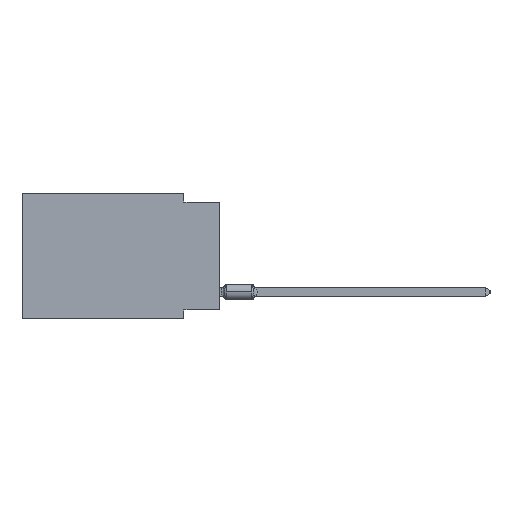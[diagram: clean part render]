
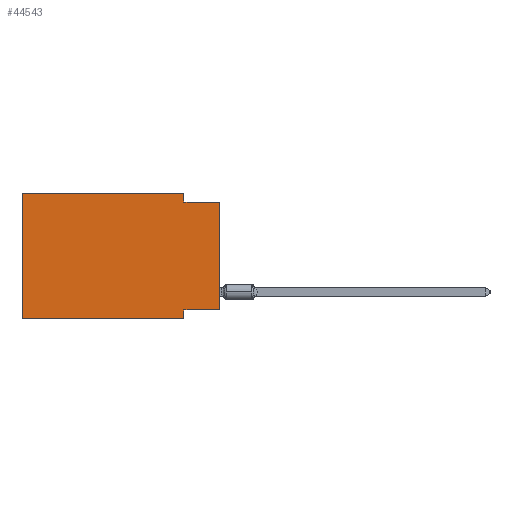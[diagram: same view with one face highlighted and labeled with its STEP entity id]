
A CAD part, left-side view. The second image highlights one B-rep face of the part: STEP entity #44543.
In plain terms, the highlighted planar face has unit normal (-1, 0, 0).
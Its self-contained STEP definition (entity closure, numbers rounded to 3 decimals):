
#1589 = VERTEX_POINT ( 'NONE', #3762 ) ;
#2478 = EDGE_CURVE ( 'NONE', #48055, #7422, #28816, .T. ) ;
#3762 = CARTESIAN_POINT ( 'NONE',  ( 0., 2.54, -8.255 ) ) ;
#4447 = EDGE_CURVE ( 'NONE', #39297, #37166, #8983, .T. ) ;
#7377 = CARTESIAN_POINT ( 'NONE',  ( 0., 2.54, -0.635 ) ) ;
#7422 = VERTEX_POINT ( 'NONE', #7377 ) ;
#7778 = DIRECTION ( 'NONE',  ( 0., -1., 0. ) ) ;
#7855 = ORIENTED_EDGE ( 'NONE', *, *, #27830, .T. ) ;
#7865 = CARTESIAN_POINT ( 'NONE',  ( 0., 0., 0. ) ) ;
#8552 = CARTESIAN_POINT ( 'NONE',  ( 0., 2.54, 0. ) ) ;
#8983 = LINE ( 'NONE', #50139, #48166 ) ;
#10203 = EDGE_CURVE ( 'NONE', #26647, #22648, #23977, .T. ) ;
#10567 = CARTESIAN_POINT ( 'NONE',  ( 0., 0., -0.635 ) ) ;
#12227 = LINE ( 'NONE', #33844, #53540 ) ;
#13186 = EDGE_LOOP ( 'NONE', ( #49338, #59941, #32141, #28366, #24407, #7855, #67055, #62164 ) ) ;
#15118 = LINE ( 'NONE', #19589, #25298 ) ;
#15498 = CARTESIAN_POINT ( 'NONE',  ( 0., 13.97, 0. ) ) ;
#15828 = PLANE ( 'NONE',  #24999 ) ;
#18811 = CARTESIAN_POINT ( 'NONE',  ( 0., 0., -0.635 ) ) ;
#19589 = CARTESIAN_POINT ( 'NONE',  ( 0., 0., -8.255 ) ) ;
#22648 = VERTEX_POINT ( 'NONE', #18811 ) ;
#23977 = LINE ( 'NONE', #7865, #40018 ) ;
#24115 = EDGE_CURVE ( 'NONE', #1589, #55991, #59589, .T. ) ;
#24407 = ORIENTED_EDGE ( 'NONE', *, *, #4447, .F. ) ;
#24999 = AXIS2_PLACEMENT_3D ( 'NONE', #15498, #36409, #58342 ) ;
#25298 = VECTOR ( 'NONE', #50462, 1000. ) ;
#26647 = VERTEX_POINT ( 'NONE', #63885 ) ;
#27830 = EDGE_CURVE ( 'NONE', #39297, #55991, #48130, .T. ) ;
#28242 = CARTESIAN_POINT ( 'NONE',  ( 0., 13.97, -8.89 ) ) ;
#28366 = ORIENTED_EDGE ( 'NONE', *, *, #62917, .F. ) ;
#28798 = DIRECTION ( 'NONE',  ( 0., 0., 1. ) ) ;
#28816 = LINE ( 'NONE', #8552, #54792 ) ;
#30902 = VECTOR ( 'NONE', #38525, 1000. ) ;
#32141 = ORIENTED_EDGE ( 'NONE', *, *, #2478, .F. ) ;
#32623 = FACE_OUTER_BOUND ( 'NONE', #13186, .T. ) ;
#33844 = CARTESIAN_POINT ( 'NONE',  ( 0., 13.97, 0. ) ) ;
#35926 = CARTESIAN_POINT ( 'NONE',  ( 0., 2.54, -8.89 ) ) ;
#36409 = DIRECTION ( 'NONE',  ( 1., 0., 0. ) ) ;
#37166 = VERTEX_POINT ( 'NONE', #62705 ) ;
#38525 = DIRECTION ( 'NONE',  ( 0., -1., 0. ) ) ;
#39297 = VERTEX_POINT ( 'NONE', #58027 ) ;
#39467 = VECTOR ( 'NONE', #63954, 1000. ) ;
#40018 = VECTOR ( 'NONE', #28798, 1000. ) ;
#42210 = CARTESIAN_POINT ( 'NONE',  ( 0., 2.54, -8.89 ) ) ;
#44070 = CARTESIAN_POINT ( 'NONE',  ( 0., 2.54, 0. ) ) ;
#44543 = ADVANCED_FACE ( 'NONE', ( #32623 ), #15828, .F. ) ;
#46920 = LINE ( 'NONE', #10567, #39467 ) ;
#47450 = EDGE_CURVE ( 'NONE', #26647, #1589, #15118, .T. ) ;
#48055 = VERTEX_POINT ( 'NONE', #44070 ) ;
#48130 = LINE ( 'NONE', #28242, #30902 ) ;
#48166 = VECTOR ( 'NONE', #60430, 1000. ) ;
#49338 = ORIENTED_EDGE ( 'NONE', *, *, #10203, .T. ) ;
#50139 = CARTESIAN_POINT ( 'NONE',  ( 0., 13.97, 0. ) ) ;
#50462 = DIRECTION ( 'NONE',  ( 0., 1., 0. ) ) ;
#51338 = VECTOR ( 'NONE', #54794, 1000. ) ;
#53540 = VECTOR ( 'NONE', #7778, 1000. ) ;
#54792 = VECTOR ( 'NONE', #59654, 1000. ) ;
#54794 = DIRECTION ( 'NONE',  ( 0., 0., -1. ) ) ;
#55991 = VERTEX_POINT ( 'NONE', #35926 ) ;
#58027 = CARTESIAN_POINT ( 'NONE',  ( 0., 13.97, -8.89 ) ) ;
#58342 = DIRECTION ( 'NONE',  ( 0., 0., -1. ) ) ;
#59589 = LINE ( 'NONE', #42210, #51338 ) ;
#59654 = DIRECTION ( 'NONE',  ( 0., 0., -1. ) ) ;
#59941 = ORIENTED_EDGE ( 'NONE', *, *, #65751, .F. ) ;
#60430 = DIRECTION ( 'NONE',  ( 0., 0., 1. ) ) ;
#62164 = ORIENTED_EDGE ( 'NONE', *, *, #47450, .F. ) ;
#62705 = CARTESIAN_POINT ( 'NONE',  ( 0., 13.97, 0. ) ) ;
#62917 = EDGE_CURVE ( 'NONE', #37166, #48055, #12227, .T. ) ;
#63885 = CARTESIAN_POINT ( 'NONE',  ( 0., 0., -8.255 ) ) ;
#63954 = DIRECTION ( 'NONE',  ( 0., -1., 0. ) ) ;
#65751 = EDGE_CURVE ( 'NONE', #7422, #22648, #46920, .T. ) ;
#67055 = ORIENTED_EDGE ( 'NONE', *, *, #24115, .F. ) ;
